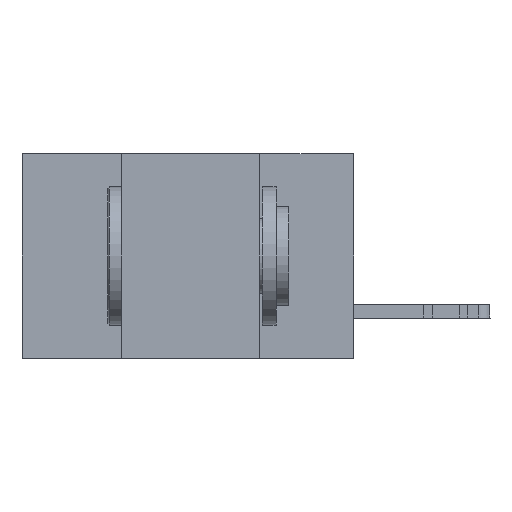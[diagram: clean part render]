
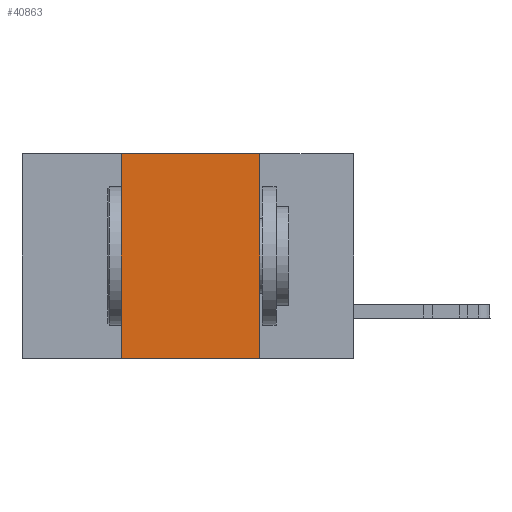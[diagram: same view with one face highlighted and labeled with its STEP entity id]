
A CAD part, left-side view. The second image highlights one B-rep face of the part: STEP entity #40863.
In plain terms, the highlighted planar face has unit normal (-1, 0, 0).
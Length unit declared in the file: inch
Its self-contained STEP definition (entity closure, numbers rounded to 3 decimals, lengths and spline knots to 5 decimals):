
#814 = FACE_OUTER_BOUND ( 'NONE', #26024, .T. ) ;
#934 = VECTOR ( 'NONE', #39810, 39.37008 ) ;
#987 = VERTEX_POINT ( 'NONE', #24533 ) ;
#1516 = CARTESIAN_POINT ( 'NONE',  ( 0., 0.6, 0. ) ) ;
#5812 = DIRECTION ( 'NONE',  ( 0., 0., 1. ) ) ;
#8006 = DIRECTION ( 'NONE',  ( 1., 0., 0. ) ) ;
#8457 = LINE ( 'NONE', #12644, #35180 ) ;
#9325 = CARTESIAN_POINT ( 'NONE',  ( 0., 0.17, 0. ) ) ;
#11409 = EDGE_CURVE ( 'NONE', #27396, #16845, #18793, .T. ) ;
#12354 = VECTOR ( 'NONE', #24840, 39.37008 ) ;
#12644 = CARTESIAN_POINT ( 'NONE',  ( 0., 0.6, 0. ) ) ;
#14983 = DIRECTION ( 'NONE',  ( 0., 0., -1. ) ) ;
#15201 = LINE ( 'NONE', #25632, #934 ) ;
#16845 = VERTEX_POINT ( 'NONE', #27058 ) ;
#18793 = LINE ( 'NONE', #29028, #12354 ) ;
#20994 = ORIENTED_EDGE ( 'NONE', *, *, #42054, .F. ) ;
#21681 = AXIS2_PLACEMENT_3D ( 'NONE', #1516, #8006, #14983 ) ;
#23110 = EDGE_CURVE ( 'NONE', #31602, #16845, #15201, .T. ) ;
#24533 = CARTESIAN_POINT ( 'NONE',  ( 0., 0.42, 0. ) ) ;
#24840 = DIRECTION ( 'NONE',  ( 0., -1., 0. ) ) ;
#25632 = CARTESIAN_POINT ( 'NONE',  ( 0., 0.17, 0. ) ) ;
#26024 = EDGE_LOOP ( 'NONE', ( #44778, #20994, #34864, #37835 ) ) ;
#27058 = CARTESIAN_POINT ( 'NONE',  ( 0., 0.17, -0.37 ) ) ;
#27396 = VERTEX_POINT ( 'NONE', #34249 ) ;
#29028 = CARTESIAN_POINT ( 'NONE',  ( 0., 0.6, -0.37 ) ) ;
#29820 = DIRECTION ( 'NONE',  ( 0., -1., 0. ) ) ;
#31602 = VERTEX_POINT ( 'NONE', #9325 ) ;
#34063 = VECTOR ( 'NONE', #5812, 39.37008 ) ;
#34249 = CARTESIAN_POINT ( 'NONE',  ( 0., 0.42, -0.37 ) ) ;
#34864 = ORIENTED_EDGE ( 'NONE', *, *, #36695, .F. ) ;
#35180 = VECTOR ( 'NONE', #29820, 39.37008 ) ;
#36695 = EDGE_CURVE ( 'NONE', #27396, #987, #41335, .T. ) ;
#37618 = CARTESIAN_POINT ( 'NONE',  ( 0., 0.42, 0. ) ) ;
#37835 = ORIENTED_EDGE ( 'NONE', *, *, #11409, .T. ) ;
#39810 = DIRECTION ( 'NONE',  ( 0., 0., -1. ) ) ;
#40863 = ADVANCED_FACE ( 'NONE', ( #814 ), #44218, .F. ) ;
#41335 = LINE ( 'NONE', #37618, #34063 ) ;
#42054 = EDGE_CURVE ( 'NONE', #987, #31602, #8457, .T. ) ;
#44218 = PLANE ( 'NONE',  #21681 ) ;
#44778 = ORIENTED_EDGE ( 'NONE', *, *, #23110, .F. ) ;
